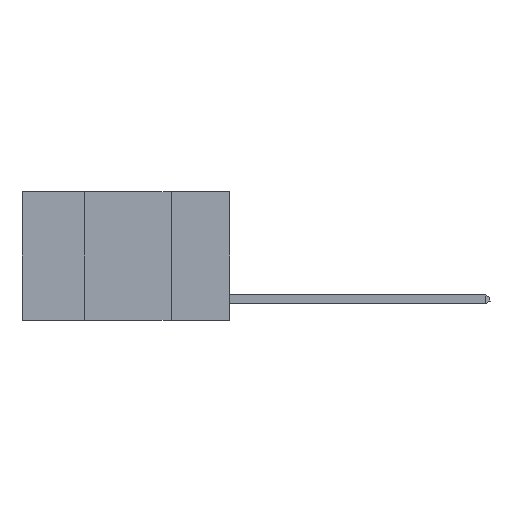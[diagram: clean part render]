
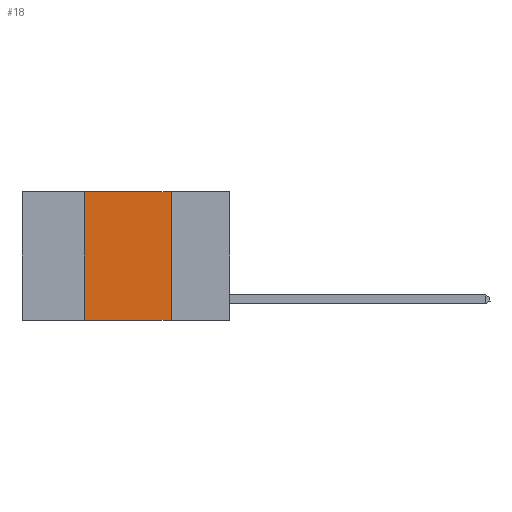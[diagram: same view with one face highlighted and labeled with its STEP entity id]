
A CAD part, left-side view. The second image highlights one B-rep face of the part: STEP entity #18.
In plain terms, the highlighted planar face has unit normal (-1, 0, 0).
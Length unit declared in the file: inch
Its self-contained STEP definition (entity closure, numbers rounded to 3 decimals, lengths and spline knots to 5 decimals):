
#18 = ADVANCED_FACE ( 'NONE', ( #15408 ), #8995, .F. ) ;
#328 = DIRECTION ( 'NONE',  ( 0., -1., 0. ) ) ;
#1261 = LINE ( 'NONE', #4767, #3869 ) ;
#1364 = CARTESIAN_POINT ( 'NONE',  ( 0., 0.42, -0.37 ) ) ;
#2120 = VERTEX_POINT ( 'NONE', #6621 ) ;
#2566 = ORIENTED_EDGE ( 'NONE', *, *, #13791, .F. ) ;
#2594 = AXIS2_PLACEMENT_3D ( 'NONE', #9491, #14115, #5123 ) ;
#2809 = CARTESIAN_POINT ( 'NONE',  ( 0., 0.17, 0. ) ) ;
#3234 = VECTOR ( 'NONE', #9080, 39.37008 ) ;
#3869 = VECTOR ( 'NONE', #13970, 39.37008 ) ;
#4619 = ORIENTED_EDGE ( 'NONE', *, *, #10496, .T. ) ;
#4767 = CARTESIAN_POINT ( 'NONE',  ( 0., 0.17, 0. ) ) ;
#5108 = CARTESIAN_POINT ( 'NONE',  ( 0., 0.6, 0. ) ) ;
#5123 = DIRECTION ( 'NONE',  ( 0., 0., -1. ) ) ;
#5985 = VERTEX_POINT ( 'NONE', #2809 ) ;
#6405 = EDGE_LOOP ( 'NONE', ( #2566, #11646, #7698, #4619 ) ) ;
#6621 = CARTESIAN_POINT ( 'NONE',  ( 0., 0.17, -0.37 ) ) ;
#6714 = CARTESIAN_POINT ( 'NONE',  ( 0., 0.6, -0.37 ) ) ;
#7698 = ORIENTED_EDGE ( 'NONE', *, *, #10443, .F. ) ;
#7784 = LINE ( 'NONE', #6714, #13262 ) ;
#8622 = EDGE_CURVE ( 'NONE', #15400, #5985, #9303, .T. ) ;
#8995 = PLANE ( 'NONE',  #2594 ) ;
#9080 = DIRECTION ( 'NONE',  ( 0., -1., 0. ) ) ;
#9303 = LINE ( 'NONE', #5108, #3234 ) ;
#9491 = CARTESIAN_POINT ( 'NONE',  ( 0., 0.6, 0. ) ) ;
#10443 = EDGE_CURVE ( 'NONE', #11781, #15400, #15287, .T. ) ;
#10496 = EDGE_CURVE ( 'NONE', #11781, #2120, #7784, .T. ) ;
#11646 = ORIENTED_EDGE ( 'NONE', *, *, #8622, .F. ) ;
#11781 = VERTEX_POINT ( 'NONE', #1364 ) ;
#12258 = VECTOR ( 'NONE', #14372, 39.37008 ) ;
#12713 = CARTESIAN_POINT ( 'NONE',  ( 0., 0.42, 0. ) ) ;
#13262 = VECTOR ( 'NONE', #328, 39.37008 ) ;
#13791 = EDGE_CURVE ( 'NONE', #5985, #2120, #1261, .T. ) ;
#13970 = DIRECTION ( 'NONE',  ( 0., 0., -1. ) ) ;
#14115 = DIRECTION ( 'NONE',  ( 1., 0., 0. ) ) ;
#14372 = DIRECTION ( 'NONE',  ( 0., 0., 1. ) ) ;
#14526 = CARTESIAN_POINT ( 'NONE',  ( 0., 0.42, 0. ) ) ;
#15287 = LINE ( 'NONE', #12713, #12258 ) ;
#15400 = VERTEX_POINT ( 'NONE', #14526 ) ;
#15408 = FACE_OUTER_BOUND ( 'NONE', #6405, .T. ) ;
